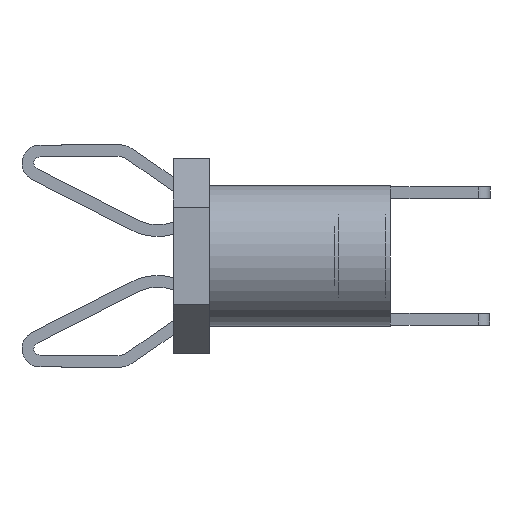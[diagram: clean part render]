
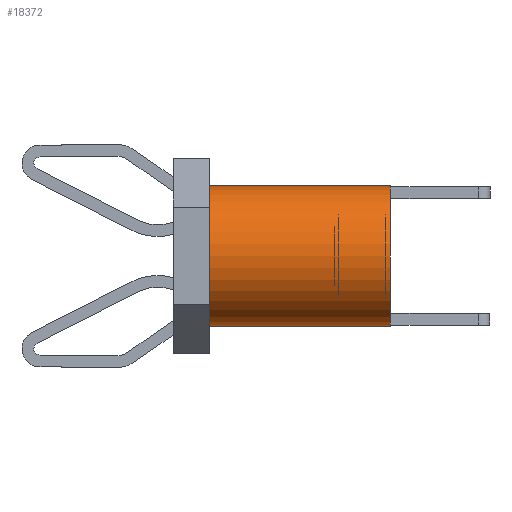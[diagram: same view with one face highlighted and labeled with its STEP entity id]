
A CAD part, left-side view. The second image highlights one B-rep face of the part: STEP entity #18372.
In plain terms, the highlighted cylindrical face has radius 1.968 mm (diameter 3.937 mm), a partial arc.
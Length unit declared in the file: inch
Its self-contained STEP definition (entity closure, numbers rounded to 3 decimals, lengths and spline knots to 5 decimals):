
#769 = EDGE_CURVE ( 'NONE', #16151, #4241, #41986, .T. ) ;
#2498 = ORIENTED_EDGE ( 'NONE', *, *, #48082, .T. ) ;
#3095 = LINE ( 'NONE', #36232, #22871 ) ;
#3288 = FACE_OUTER_BOUND ( 'NONE', #19815, .T. ) ;
#3771 = CIRCLE ( 'NONE', #31802, 0.0775 ) ;
#4241 = VERTEX_POINT ( 'NONE', #41293 ) ;
#4279 = VERTEX_POINT ( 'NONE', #41459 ) ;
#4834 = VERTEX_POINT ( 'NONE', #30119 ) ;
#5469 = DIRECTION ( 'NONE',  ( 0., -1., 0. ) ) ;
#6928 = AXIS2_PLACEMENT_3D ( 'NONE', #10752, #38230, #14697 ) ;
#7808 = ORIENTED_EDGE ( 'NONE', *, *, #27932, .T. ) ;
#9429 = DIRECTION ( 'NONE',  ( 0., 1., 0. ) ) ;
#10752 = CARTESIAN_POINT ( 'NONE',  ( 0., 0.24, 0. ) ) ;
#14697 = DIRECTION ( 'NONE',  ( 0., 0., 1. ) ) ;
#16151 = VERTEX_POINT ( 'NONE', #49436 ) ;
#17376 = DIRECTION ( 'NONE',  ( 0., 0., -1. ) ) ;
#18372 = ADVANCED_FACE ( 'NONE', ( #3288 ), #33476, .T. ) ;
#18630 = CARTESIAN_POINT ( 'NONE',  ( 0., 0.24, 0.0775 ) ) ;
#19815 = EDGE_LOOP ( 'NONE', ( #29234, #40084, #7808, #2498 ) ) ;
#22871 = VECTOR ( 'NONE', #48183, 39.37008 ) ;
#27932 = EDGE_CURVE ( 'NONE', #4834, #4279, #3095, .T. ) ;
#29171 = VECTOR ( 'NONE', #49769, 39.37008 ) ;
#29234 = ORIENTED_EDGE ( 'NONE', *, *, #769, .F. ) ;
#30119 = CARTESIAN_POINT ( 'NONE',  ( 0., 0.24, -0.0775 ) ) ;
#31802 = AXIS2_PLACEMENT_3D ( 'NONE', #32982, #9429, #36911 ) ;
#32982 = CARTESIAN_POINT ( 'NONE',  ( 0., 0.04, 0. ) ) ;
#33476 = CYLINDRICAL_SURFACE ( 'NONE', #48543, 0.0775 ) ;
#36232 = CARTESIAN_POINT ( 'NONE',  ( 0., 0.24, -0.0775 ) ) ;
#36911 = DIRECTION ( 'NONE',  ( 0., 0., 1. ) ) ;
#38230 = DIRECTION ( 'NONE',  ( 0., 1., 0. ) ) ;
#40084 = ORIENTED_EDGE ( 'NONE', *, *, #43707, .F. ) ;
#40866 = CARTESIAN_POINT ( 'NONE',  ( 0., 0.24, 0. ) ) ;
#41293 = CARTESIAN_POINT ( 'NONE',  ( 0., 0.04, 0.0775 ) ) ;
#41459 = CARTESIAN_POINT ( 'NONE',  ( 0., 0.04, -0.0775 ) ) ;
#41986 = LINE ( 'NONE', #18630, #29171 ) ;
#43707 = EDGE_CURVE ( 'NONE', #4834, #16151, #45907, .T. ) ;
#45907 = CIRCLE ( 'NONE', #6928, 0.0775 ) ;
#48082 = EDGE_CURVE ( 'NONE', #4279, #4241, #3771, .T. ) ;
#48183 = DIRECTION ( 'NONE',  ( 0., -1., 0. ) ) ;
#48543 = AXIS2_PLACEMENT_3D ( 'NONE', #40866, #5469, #17376 ) ;
#49436 = CARTESIAN_POINT ( 'NONE',  ( 0., 0.24, 0.0775 ) ) ;
#49769 = DIRECTION ( 'NONE',  ( 0., -1., 0. ) ) ;
